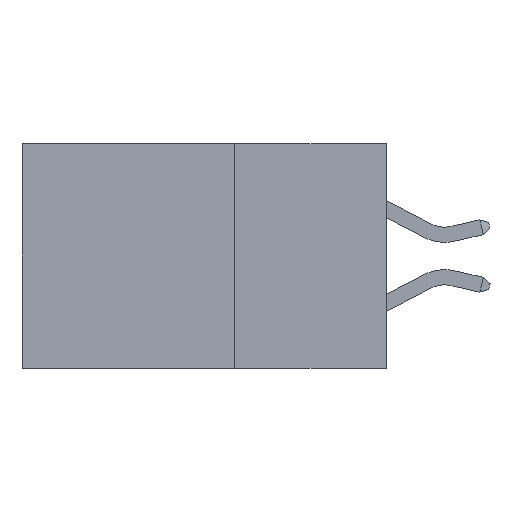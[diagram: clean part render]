
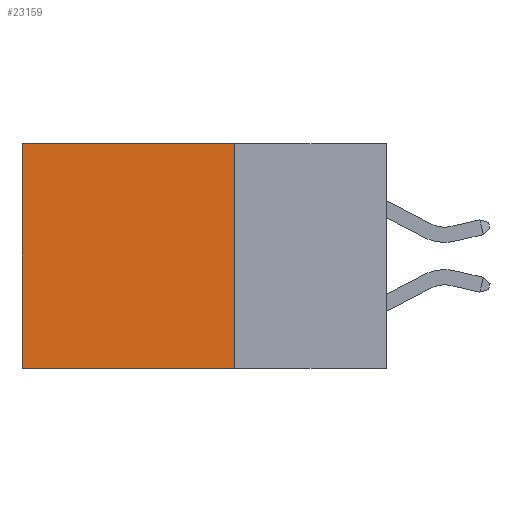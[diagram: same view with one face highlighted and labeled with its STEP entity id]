
A CAD part, left-side view. The second image highlights one B-rep face of the part: STEP entity #23159.
In plain terms, the highlighted planar face has unit normal (-1, 0, 0).
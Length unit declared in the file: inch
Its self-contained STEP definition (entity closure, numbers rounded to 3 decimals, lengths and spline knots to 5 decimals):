
#608 = DIRECTION ( 'NONE',  ( 0., 1., 0. ) ) ;
#2580 = LINE ( 'NONE', #23195, #3839 ) ;
#3439 = ORIENTED_EDGE ( 'NONE', *, *, #19934, .F. ) ;
#3839 = VECTOR ( 'NONE', #15191, 39.37008 ) ;
#5833 = EDGE_CURVE ( 'NONE', #8465, #12698, #2580, .T. ) ;
#6196 = CARTESIAN_POINT ( 'NONE',  ( 0.298, 0.6, 0. ) ) ;
#8465 = VERTEX_POINT ( 'NONE', #9239 ) ;
#8672 = DIRECTION ( 'NONE',  ( 0., 0., -1. ) ) ;
#9239 = CARTESIAN_POINT ( 'NONE',  ( 0.298, 0.25, -0.37 ) ) ;
#9248 = VECTOR ( 'NONE', #20534, 39.37008 ) ;
#10916 = VECTOR ( 'NONE', #608, 39.37008 ) ;
#11309 = ORIENTED_EDGE ( 'NONE', *, *, #16835, .T. ) ;
#11569 = FACE_OUTER_BOUND ( 'NONE', #12238, .T. ) ;
#11664 = PLANE ( 'NONE',  #12240 ) ;
#11740 = CARTESIAN_POINT ( 'NONE',  ( 0.298, 0.6, -0.37 ) ) ;
#11770 = VECTOR ( 'NONE', #8672, 39.37008 ) ;
#11997 = CARTESIAN_POINT ( 'NONE',  ( 0.298, 0.25, 0. ) ) ;
#12238 = EDGE_LOOP ( 'NONE', ( #11309, #19549, #3439, #21363 ) ) ;
#12240 = AXIS2_PLACEMENT_3D ( 'NONE', #22118, #24177, #13624 ) ;
#12698 = VERTEX_POINT ( 'NONE', #11740 ) ;
#13624 = DIRECTION ( 'NONE',  ( 0., 0., -1. ) ) ;
#14685 = CARTESIAN_POINT ( 'NONE',  ( 0.298, 0.25, 0. ) ) ;
#15191 = DIRECTION ( 'NONE',  ( 0., 1., 0. ) ) ;
#16247 = LINE ( 'NONE', #14685, #9248 ) ;
#16271 = CARTESIAN_POINT ( 'NONE',  ( 0.298, 0.25, 0. ) ) ;
#16835 = EDGE_CURVE ( 'NONE', #18053, #12698, #19055, .T. ) ;
#17273 = LINE ( 'NONE', #16271, #10916 ) ;
#18053 = VERTEX_POINT ( 'NONE', #6196 ) ;
#19055 = LINE ( 'NONE', #20845, #11770 ) ;
#19486 = VERTEX_POINT ( 'NONE', #11997 ) ;
#19549 = ORIENTED_EDGE ( 'NONE', *, *, #5833, .F. ) ;
#19934 = EDGE_CURVE ( 'NONE', #19486, #8465, #16247, .T. ) ;
#20534 = DIRECTION ( 'NONE',  ( 0., 0., -1. ) ) ;
#20845 = CARTESIAN_POINT ( 'NONE',  ( 0.298, 0.6, 0. ) ) ;
#21363 = ORIENTED_EDGE ( 'NONE', *, *, #23383, .T. ) ;
#22118 = CARTESIAN_POINT ( 'NONE',  ( 0.298, 0.25, 0. ) ) ;
#23159 = ADVANCED_FACE ( 'NONE', ( #11569 ), #11664, .F. ) ;
#23195 = CARTESIAN_POINT ( 'NONE',  ( 0.298, 0.25, -0.37 ) ) ;
#23383 = EDGE_CURVE ( 'NONE', #19486, #18053, #17273, .T. ) ;
#24177 = DIRECTION ( 'NONE',  ( 1., 0., 0. ) ) ;
